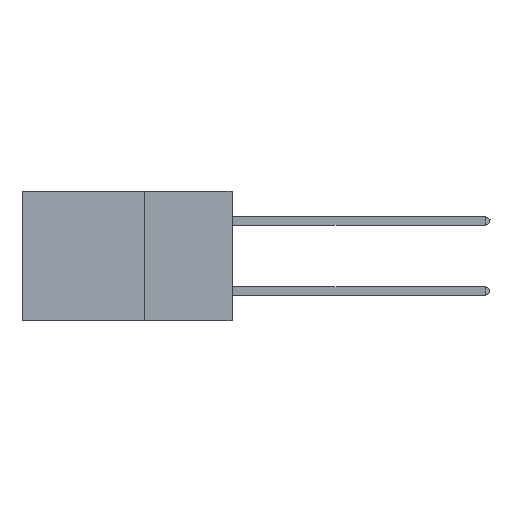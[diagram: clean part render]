
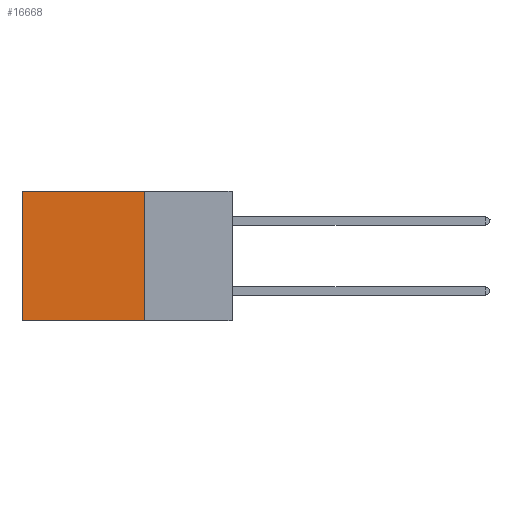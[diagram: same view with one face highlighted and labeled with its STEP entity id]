
A CAD part, left-side view. The second image highlights one B-rep face of the part: STEP entity #16668.
In plain terms, the highlighted planar face has unit normal (-1, 0, 0).
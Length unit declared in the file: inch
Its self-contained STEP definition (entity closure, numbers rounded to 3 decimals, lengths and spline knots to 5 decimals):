
#307 = DIRECTION ( 'NONE',  ( 0., 1., 0. ) ) ;
#558 = DIRECTION ( 'NONE',  ( 1., 0., 0. ) ) ;
#2843 = VERTEX_POINT ( 'NONE', #35343 ) ;
#3705 = ORIENTED_EDGE ( 'NONE', *, *, #27903, .F. ) ;
#5651 = LINE ( 'NONE', #42197, #6940 ) ;
#6940 = VECTOR ( 'NONE', #27741, 39.37008 ) ;
#7428 = EDGE_CURVE ( 'NONE', #2843, #7616, #14773, .T. ) ;
#7532 = CARTESIAN_POINT ( 'NONE',  ( 0.2875, 0.25, -0.37 ) ) ;
#7616 = VERTEX_POINT ( 'NONE', #13534 ) ;
#11888 = CARTESIAN_POINT ( 'NONE',  ( 0.2875, 0.25, 0. ) ) ;
#13534 = CARTESIAN_POINT ( 'NONE',  ( 0.2875, 0.6, 0. ) ) ;
#14173 = EDGE_CURVE ( 'NONE', #2843, #45498, #42080, .T. ) ;
#14773 = LINE ( 'NONE', #11888, #29389 ) ;
#14957 = LINE ( 'NONE', #7532, #20089 ) ;
#16668 = ADVANCED_FACE ( 'NONE', ( #18576 ), #21700, .F. ) ;
#18576 = FACE_OUTER_BOUND ( 'NONE', #33379, .T. ) ;
#19477 = CARTESIAN_POINT ( 'NONE',  ( 0.2875, 0.25, 0. ) ) ;
#20089 = VECTOR ( 'NONE', #307, 39.37008 ) ;
#21700 = PLANE ( 'NONE',  #37631 ) ;
#22632 = CARTESIAN_POINT ( 'NONE',  ( 0.2875, 0.25, 0. ) ) ;
#25292 = DIRECTION ( 'NONE',  ( 0., 0., -1. ) ) ;
#27248 = VERTEX_POINT ( 'NONE', #38379 ) ;
#27741 = DIRECTION ( 'NONE',  ( 0., 0., -1. ) ) ;
#27903 = EDGE_CURVE ( 'NONE', #45498, #27248, #14957, .T. ) ;
#29389 = VECTOR ( 'NONE', #32808, 39.37008 ) ;
#30538 = DIRECTION ( 'NONE',  ( 0., 0., -1. ) ) ;
#30969 = ORIENTED_EDGE ( 'NONE', *, *, #7428, .T. ) ;
#32808 = DIRECTION ( 'NONE',  ( 0., 1., 0. ) ) ;
#33379 = EDGE_LOOP ( 'NONE', ( #45950, #3705, #41507, #30969 ) ) ;
#35343 = CARTESIAN_POINT ( 'NONE',  ( 0.2875, 0.25, 0. ) ) ;
#37631 = AXIS2_PLACEMENT_3D ( 'NONE', #22632, #558, #25292 ) ;
#38379 = CARTESIAN_POINT ( 'NONE',  ( 0.2875, 0.6, -0.37 ) ) ;
#39473 = CARTESIAN_POINT ( 'NONE',  ( 0.2875, 0.25, -0.37 ) ) ;
#41507 = ORIENTED_EDGE ( 'NONE', *, *, #14173, .F. ) ;
#42080 = LINE ( 'NONE', #19477, #46683 ) ;
#42197 = CARTESIAN_POINT ( 'NONE',  ( 0.2875, 0.6, 0. ) ) ;
#45498 = VERTEX_POINT ( 'NONE', #39473 ) ;
#45950 = ORIENTED_EDGE ( 'NONE', *, *, #46569, .T. ) ;
#46569 = EDGE_CURVE ( 'NONE', #7616, #27248, #5651, .T. ) ;
#46683 = VECTOR ( 'NONE', #30538, 39.37008 ) ;
